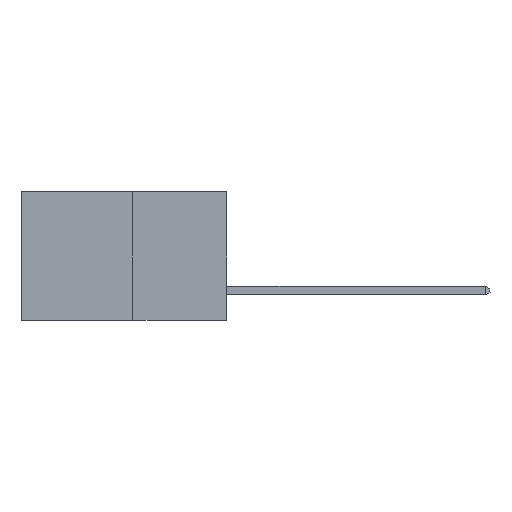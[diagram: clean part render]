
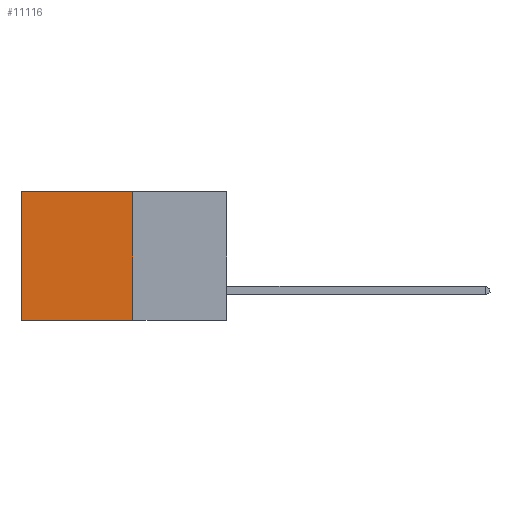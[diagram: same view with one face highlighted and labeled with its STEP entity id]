
A CAD part, left-side view. The second image highlights one B-rep face of the part: STEP entity #11116.
In plain terms, the highlighted planar face has unit normal (-1, 0, 0).
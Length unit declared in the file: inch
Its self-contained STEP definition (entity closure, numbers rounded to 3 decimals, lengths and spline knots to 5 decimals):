
#387 = DIRECTION ( 'NONE',  ( 0., 1., 0. ) ) ;
#2850 = VECTOR ( 'NONE', #387, 39.37008 ) ;
#3061 = EDGE_CURVE ( 'NONE', #5372, #7318, #7597, .T. ) ;
#3121 = VERTEX_POINT ( 'NONE', #9175 ) ;
#3770 = VERTEX_POINT ( 'NONE', #16793 ) ;
#4359 = AXIS2_PLACEMENT_3D ( 'NONE', #6474, #17732, #9318 ) ;
#5047 = PLANE ( 'NONE',  #4359 ) ;
#5372 = VERTEX_POINT ( 'NONE', #10048 ) ;
#6269 = ORIENTED_EDGE ( 'NONE', *, *, #6508, .T. ) ;
#6407 = ORIENTED_EDGE ( 'NONE', *, *, #15709, .F. ) ;
#6474 = CARTESIAN_POINT ( 'NONE',  ( 0.277, 0.27, -0.37 ) ) ;
#6508 = EDGE_CURVE ( 'NONE', #7318, #3121, #18223, .T. ) ;
#7155 = VECTOR ( 'NONE', #9677, 39.37008 ) ;
#7318 = VERTEX_POINT ( 'NONE', #14443 ) ;
#7597 = LINE ( 'NONE', #15430, #7155 ) ;
#8857 = VECTOR ( 'NONE', #16866, 39.37008 ) ;
#9175 = CARTESIAN_POINT ( 'NONE',  ( 0.277, 0.59, -0.37 ) ) ;
#9318 = DIRECTION ( 'NONE',  ( 0., 0., -1. ) ) ;
#9677 = DIRECTION ( 'NONE',  ( 0., 1., 0. ) ) ;
#9895 = CARTESIAN_POINT ( 'NONE',  ( 0.277, 0.27, -0.37 ) ) ;
#10048 = CARTESIAN_POINT ( 'NONE',  ( 0.277, 0.27, 0. ) ) ;
#10343 = CARTESIAN_POINT ( 'NONE',  ( 0.277, 0.27, -0.37 ) ) ;
#10413 = LINE ( 'NONE', #10343, #2850 ) ;
#11116 = ADVANCED_FACE ( 'NONE', ( #16939 ), #5047, .F. ) ;
#12737 = ORIENTED_EDGE ( 'NONE', *, *, #3061, .T. ) ;
#12821 = CARTESIAN_POINT ( 'NONE',  ( 0.277, 0.59, -0.37 ) ) ;
#12873 = DIRECTION ( 'NONE',  ( 0., 0., -1. ) ) ;
#13078 = LINE ( 'NONE', #9895, #8857 ) ;
#14443 = CARTESIAN_POINT ( 'NONE',  ( 0.277, 0.59, 0. ) ) ;
#14445 = ORIENTED_EDGE ( 'NONE', *, *, #16672, .F. ) ;
#15379 = VECTOR ( 'NONE', #12873, 39.37008 ) ;
#15430 = CARTESIAN_POINT ( 'NONE',  ( 0.277, 0.27, 0. ) ) ;
#15709 = EDGE_CURVE ( 'NONE', #5372, #3770, #13078, .T. ) ;
#16377 = EDGE_LOOP ( 'NONE', ( #6269, #14445, #6407, #12737 ) ) ;
#16672 = EDGE_CURVE ( 'NONE', #3770, #3121, #10413, .T. ) ;
#16793 = CARTESIAN_POINT ( 'NONE',  ( 0.277, 0.27, -0.37 ) ) ;
#16866 = DIRECTION ( 'NONE',  ( 0., 0., -1. ) ) ;
#16939 = FACE_OUTER_BOUND ( 'NONE', #16377, .T. ) ;
#17732 = DIRECTION ( 'NONE',  ( 1., 0., 0. ) ) ;
#18223 = LINE ( 'NONE', #12821, #15379 ) ;
